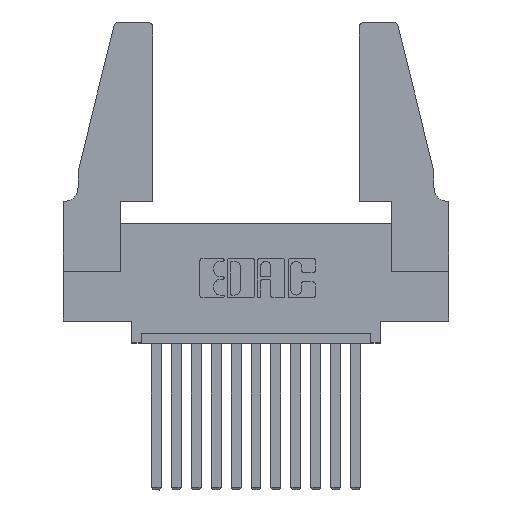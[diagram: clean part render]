
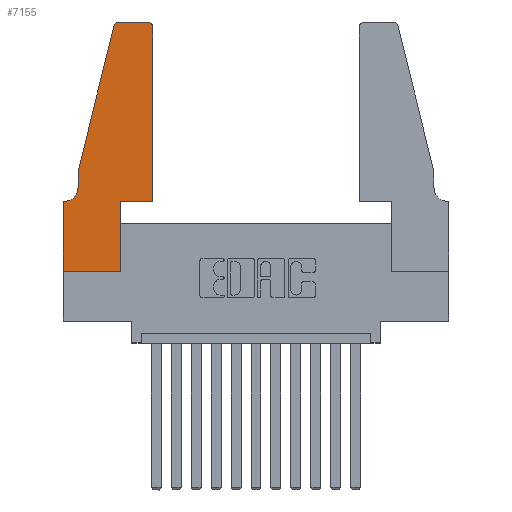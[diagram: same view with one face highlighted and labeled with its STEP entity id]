
A CAD part, top view. The second image highlights one B-rep face of the part: STEP entity #7155.
In plain terms, the highlighted planar face has unit normal (0, 0, 1).
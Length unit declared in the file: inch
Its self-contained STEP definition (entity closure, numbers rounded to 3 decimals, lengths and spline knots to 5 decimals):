
#53 = CARTESIAN_POINT ( 'NONE',  ( 0.0755, 0.35, 0.37 ) ) ;
#57 = LINE ( 'NONE', #3885, #12166 ) ;
#109 = LINE ( 'NONE', #4915, #631 ) ;
#466 = AXIS2_PLACEMENT_3D ( 'NONE', #5086, #5034, #8479 ) ;
#605 = CARTESIAN_POINT ( 'NONE',  ( 0., 0., 0.37 ) ) ;
#631 = VECTOR ( 'NONE', #9680, 39.37008 ) ;
#663 = VECTOR ( 'NONE', #2473, 39.37008 ) ;
#689 = DIRECTION ( 'NONE',  ( 0., 0., 1. ) ) ;
#893 = ORIENTED_EDGE ( 'NONE', *, *, #5817, .T. ) ;
#1241 = LINE ( 'NONE', #3331, #5440 ) ;
#1693 = CARTESIAN_POINT ( 'NONE',  ( 0.4505, 0.35, 0.37 ) ) ;
#1781 = CARTESIAN_POINT ( 'NONE',  ( 0.4205, 1.25, 0.37 ) ) ;
#1813 = DIRECTION ( 'NONE',  ( 0., 0., 1. ) ) ;
#1866 = LINE ( 'NONE', #5650, #4811 ) ;
#2154 = EDGE_CURVE ( 'NONE', #2974, #5869, #8609, .T. ) ;
#2410 = CIRCLE ( 'NONE', #466, 0.03 ) ;
#2473 = DIRECTION ( 'NONE',  ( 0., -1., 0. ) ) ;
#2480 = ORIENTED_EDGE ( 'NONE', *, *, #8344, .T. ) ;
#2592 = CARTESIAN_POINT ( 'NONE',  ( 0.2865, 0., 0.37 ) ) ;
#2727 = VERTEX_POINT ( 'NONE', #1693 ) ;
#2904 = VERTEX_POINT ( 'NONE', #7051 ) ;
#2974 = VERTEX_POINT ( 'NONE', #5956 ) ;
#3113 = EDGE_CURVE ( 'NONE', #12601, #6566, #9204, .T. ) ;
#3298 = AXIS2_PLACEMENT_3D ( 'NONE', #13124, #13068, #13176 ) ;
#3331 = CARTESIAN_POINT ( 'NONE',  ( 0.4505, 0.35, 0.37 ) ) ;
#3609 = ORIENTED_EDGE ( 'NONE', *, *, #10127, .T. ) ;
#3617 = CARTESIAN_POINT ( 'NONE',  ( 0., 0.35, 0.37 ) ) ;
#3885 = CARTESIAN_POINT ( 'NONE',  ( 0., 0., 0.37 ) ) ;
#3914 = VERTEX_POINT ( 'NONE', #7018 ) ;
#4237 = AXIS2_PLACEMENT_3D ( 'NONE', #14152, #689, #6617 ) ;
#4369 = EDGE_CURVE ( 'NONE', #13896, #2727, #1241, .T. ) ;
#4424 = AXIS2_PLACEMENT_3D ( 'NONE', #5129, #1813, #14186 ) ;
#4811 = VECTOR ( 'NONE', #13285, 39.37008 ) ;
#4915 = CARTESIAN_POINT ( 'NONE',  ( 0.2865, 0.35, 0.37 ) ) ;
#5034 = DIRECTION ( 'NONE',  ( 0., 0., 1. ) ) ;
#5086 = CARTESIAN_POINT ( 'NONE',  ( 0.284, 1.22, 0.37 ) ) ;
#5129 = CARTESIAN_POINT ( 'NONE',  ( 0., 0.35, 0.37 ) ) ;
#5209 = LINE ( 'NONE', #5783, #663 ) ;
#5222 = CIRCLE ( 'NONE', #4237, 0.03 ) ;
#5419 = VERTEX_POINT ( 'NONE', #605 ) ;
#5440 = VECTOR ( 'NONE', #10761, 39.37008 ) ;
#5567 = VECTOR ( 'NONE', #13789, 39.37008 ) ;
#5571 = ORIENTED_EDGE ( 'NONE', *, *, #11670, .T. ) ;
#5616 = VECTOR ( 'NONE', #7723, 39.37008 ) ;
#5624 = VERTEX_POINT ( 'NONE', #1781 ) ;
#5650 = CARTESIAN_POINT ( 'NONE',  ( 0.0755, 0.5, 0.37 ) ) ;
#5778 = CARTESIAN_POINT ( 'NONE',  ( 0.4505, 0.35, 0.37 ) ) ;
#5783 = CARTESIAN_POINT ( 'NONE',  ( 0., 0., 0.37 ) ) ;
#5817 = EDGE_CURVE ( 'NONE', #2904, #5624, #5222, .T. ) ;
#5869 = VERTEX_POINT ( 'NONE', #9656 ) ;
#5956 = CARTESIAN_POINT ( 'NONE',  ( 0.25487, 1.22718, 0.37 ) ) ;
#6071 = FACE_OUTER_BOUND ( 'NONE', #6689, .T. ) ;
#6427 = ORIENTED_EDGE ( 'NONE', *, *, #6697, .T. ) ;
#6552 = EDGE_CURVE ( 'NONE', #2727, #2904, #8758, .T. ) ;
#6566 = VERTEX_POINT ( 'NONE', #3617 ) ;
#6616 = EDGE_CURVE ( 'NONE', #12563, #2974, #2410, .T. ) ;
#6617 = DIRECTION ( 'NONE',  ( 1., 0., 0. ) ) ;
#6689 = EDGE_LOOP ( 'NONE', ( #3609, #12898, #13715, #11457, #6427, #7813, #5571, #2480, #14486, #14503, #10951, #893 ) ) ;
#6697 = EDGE_CURVE ( 'NONE', #3914, #12601, #12559, .T. ) ;
#7018 = CARTESIAN_POINT ( 'NONE',  ( 0.0755, 0.42, 0.37 ) ) ;
#7051 = CARTESIAN_POINT ( 'NONE',  ( 0.4505, 1.22, 0.37 ) ) ;
#7155 = ADVANCED_FACE ( 'NONE', ( #6071 ), #10805, .T. ) ;
#7402 = EDGE_CURVE ( 'NONE', #5869, #3914, #1866, .T. ) ;
#7723 = DIRECTION ( 'NONE',  ( -1., 0., 0. ) ) ;
#7813 = ORIENTED_EDGE ( 'NONE', *, *, #3113, .T. ) ;
#7868 = CARTESIAN_POINT ( 'NONE',  ( 0.2605, 1.25, 0.37 ) ) ;
#8344 = EDGE_CURVE ( 'NONE', #5419, #10353, #57, .T. ) ;
#8479 = DIRECTION ( 'NONE',  ( 1., 0., 0. ) ) ;
#8609 = LINE ( 'NONE', #10557, #5567 ) ;
#8758 = LINE ( 'NONE', #5778, #11052 ) ;
#9120 = CARTESIAN_POINT ( 'NONE',  ( 0.2865, 0.35, 0.37 ) ) ;
#9204 = LINE ( 'NONE', #53, #9725 ) ;
#9656 = CARTESIAN_POINT ( 'NONE',  ( 0.0755, 0.5, 0.37 ) ) ;
#9680 = DIRECTION ( 'NONE',  ( 0., 1., 0. ) ) ;
#9725 = VECTOR ( 'NONE', #10201, 39.37008 ) ;
#9947 = CARTESIAN_POINT ( 'NONE',  ( 0.284, 1.25, 0.37 ) ) ;
#10127 = EDGE_CURVE ( 'NONE', #5624, #12563, #13022, .T. ) ;
#10182 = CARTESIAN_POINT ( 'NONE',  ( 0.0055, 0.35, 0.37 ) ) ;
#10201 = DIRECTION ( 'NONE',  ( -1., 0., 0. ) ) ;
#10345 = DIRECTION ( 'NONE',  ( 0., 1., 0. ) ) ;
#10353 = VERTEX_POINT ( 'NONE', #2592 ) ;
#10557 = CARTESIAN_POINT ( 'NONE',  ( 0.0755, 0.5, 0.37 ) ) ;
#10761 = DIRECTION ( 'NONE',  ( 1., 0., 0. ) ) ;
#10805 = PLANE ( 'NONE',  #4424 ) ;
#10951 = ORIENTED_EDGE ( 'NONE', *, *, #6552, .T. ) ;
#11052 = VECTOR ( 'NONE', #10345, 39.37008 ) ;
#11457 = ORIENTED_EDGE ( 'NONE', *, *, #7402, .T. ) ;
#11670 = EDGE_CURVE ( 'NONE', #6566, #5419, #5209, .T. ) ;
#12166 = VECTOR ( 'NONE', #12943, 39.37008 ) ;
#12559 = CIRCLE ( 'NONE', #3298, 0.07 ) ;
#12563 = VERTEX_POINT ( 'NONE', #9947 ) ;
#12601 = VERTEX_POINT ( 'NONE', #10182 ) ;
#12898 = ORIENTED_EDGE ( 'NONE', *, *, #6616, .T. ) ;
#12943 = DIRECTION ( 'NONE',  ( 1., 0., 0. ) ) ;
#13013 = EDGE_CURVE ( 'NONE', #10353, #13896, #109, .T. ) ;
#13022 = LINE ( 'NONE', #7868, #5616 ) ;
#13068 = DIRECTION ( 'NONE',  ( 0., 0., -1. ) ) ;
#13124 = CARTESIAN_POINT ( 'NONE',  ( 0.0055, 0.42, 0.37 ) ) ;
#13176 = DIRECTION ( 'NONE',  ( -1., 0., 0. ) ) ;
#13285 = DIRECTION ( 'NONE',  ( 0., -1., 0. ) ) ;
#13715 = ORIENTED_EDGE ( 'NONE', *, *, #2154, .T. ) ;
#13789 = DIRECTION ( 'NONE',  ( -0.239, -0.971, 0. ) ) ;
#13896 = VERTEX_POINT ( 'NONE', #9120 ) ;
#14152 = CARTESIAN_POINT ( 'NONE',  ( 0.4205, 1.22, 0.37 ) ) ;
#14186 = DIRECTION ( 'NONE',  ( 1., 0., 0. ) ) ;
#14486 = ORIENTED_EDGE ( 'NONE', *, *, #13013, .T. ) ;
#14503 = ORIENTED_EDGE ( 'NONE', *, *, #4369, .T. ) ;
